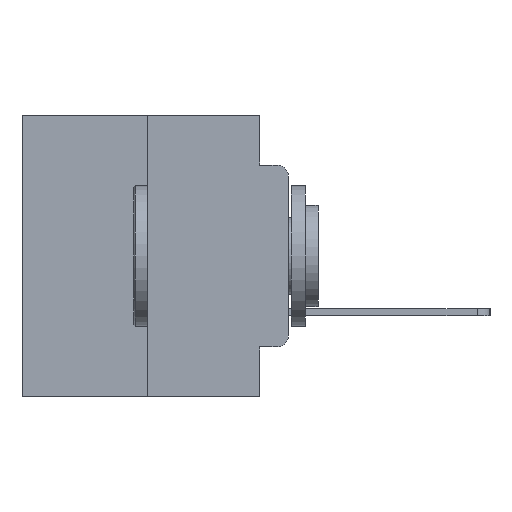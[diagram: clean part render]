
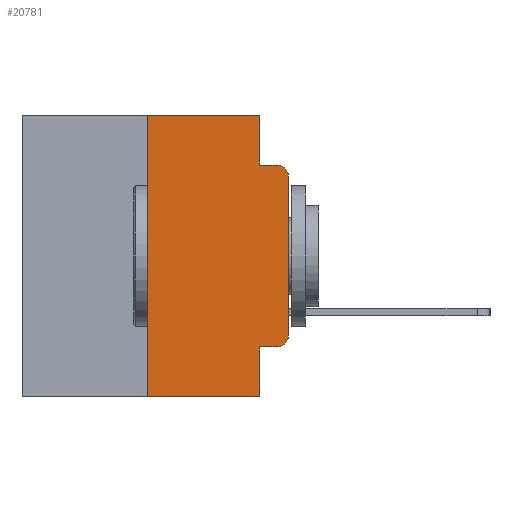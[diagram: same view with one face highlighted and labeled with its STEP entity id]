
A CAD part, left-side view. The second image highlights one B-rep face of the part: STEP entity #20781.
In plain terms, the highlighted planar face has unit normal (-1, 0, 0).
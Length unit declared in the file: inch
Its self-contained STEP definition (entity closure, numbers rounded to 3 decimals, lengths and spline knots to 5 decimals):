
#419 = EDGE_CURVE ( 'NONE', #8663, #21818, #3495, .T. ) ;
#1797 = ORIENTED_EDGE ( 'NONE', *, *, #419, .T. ) ;
#1842 = AXIS2_PLACEMENT_3D ( 'NONE', #24012, #11485, #26080 ) ;
#2052 = PLANE ( 'NONE',  #5337 ) ;
#2612 = VECTOR ( 'NONE', #22174, 39.37008 ) ;
#3182 = CARTESIAN_POINT ( 'NONE',  ( 0., 0.051, 0. ) ) ;
#3195 = CARTESIAN_POINT ( 'NONE',  ( 0., 0.473, 0. ) ) ;
#3435 = VERTEX_POINT ( 'NONE', #15398 ) ;
#3495 = LINE ( 'NONE', #5532, #24544 ) ;
#3558 = EDGE_CURVE ( 'NONE', #20752, #16808, #25629, .T. ) ;
#3563 = CARTESIAN_POINT ( 'NONE',  ( 0., 0.25, -0.5 ) ) ;
#3570 = CIRCLE ( 'NONE', #1842, 0.02 ) ;
#3607 = LINE ( 'NONE', #26743, #25941 ) ;
#3719 = EDGE_CURVE ( 'NONE', #14574, #13075, #3607, .T. ) ;
#3891 = ORIENTED_EDGE ( 'NONE', *, *, #3558, .F. ) ;
#4219 = ORIENTED_EDGE ( 'NONE', *, *, #25009, .F. ) ;
#4962 = VECTOR ( 'NONE', #10545, 39.37008 ) ;
#5025 = DIRECTION ( 'NONE',  ( 0., 0., -1. ) ) ;
#5337 = AXIS2_PLACEMENT_3D ( 'NONE', #10537, #25245, #12712 ) ;
#5505 = VECTOR ( 'NONE', #20684, 39.37008 ) ;
#5532 = CARTESIAN_POINT ( 'NONE',  ( 0., 0., 0. ) ) ;
#6277 = CARTESIAN_POINT ( 'NONE',  ( 0., 0.051, -0.0885 ) ) ;
#6573 = ORIENTED_EDGE ( 'NONE', *, *, #3719, .T. ) ;
#7925 = ORIENTED_EDGE ( 'NONE', *, *, #10982, .T. ) ;
#8055 = LINE ( 'NONE', #13450, #12942 ) ;
#8663 = VERTEX_POINT ( 'NONE', #10438 ) ;
#8932 = CIRCLE ( 'NONE', #16499, 0.02 ) ;
#8959 = DIRECTION ( 'NONE',  ( 0., 0., -1. ) ) ;
#9341 = LINE ( 'NONE', #19435, #14285 ) ;
#9593 = EDGE_CURVE ( 'NONE', #3435, #8663, #8932, .T. ) ;
#9643 = CARTESIAN_POINT ( 'NONE',  ( 0., 0.051, -0.0885 ) ) ;
#9742 = LINE ( 'NONE', #13817, #20249 ) ;
#9857 = CARTESIAN_POINT ( 'NONE',  ( 0., 0.02, -0.3915 ) ) ;
#10438 = CARTESIAN_POINT ( 'NONE',  ( 0., 0., -0.3915 ) ) ;
#10537 = CARTESIAN_POINT ( 'NONE',  ( 0., 0.473, 0. ) ) ;
#10545 = DIRECTION ( 'NONE',  ( 0., -1., 0. ) ) ;
#10982 = EDGE_CURVE ( 'NONE', #21681, #3435, #11123, .T. ) ;
#11123 = LINE ( 'NONE', #12231, #5505 ) ;
#11267 = LINE ( 'NONE', #6277, #4962 ) ;
#11485 = DIRECTION ( 'NONE',  ( -1., 0., 0. ) ) ;
#11933 = DIRECTION ( 'NONE',  ( 0., 0., -1. ) ) ;
#12160 = DIRECTION ( 'NONE',  ( 0., -1., 0. ) ) ;
#12231 = CARTESIAN_POINT ( 'NONE',  ( 0., 0.051, -0.4115 ) ) ;
#12712 = DIRECTION ( 'NONE',  ( 0., 0., -1. ) ) ;
#12942 = VECTOR ( 'NONE', #5025, 39.37008 ) ;
#13075 = VERTEX_POINT ( 'NONE', #21981 ) ;
#13450 = CARTESIAN_POINT ( 'NONE',  ( 0., 0.051, 0. ) ) ;
#13817 = CARTESIAN_POINT ( 'NONE',  ( 0., 0.25, 0. ) ) ;
#14285 = VECTOR ( 'NONE', #8959, 39.37008 ) ;
#14574 = VERTEX_POINT ( 'NONE', #3563 ) ;
#15398 = CARTESIAN_POINT ( 'NONE',  ( 0., 0.02, -0.4115 ) ) ;
#15904 = DIRECTION ( 'NONE',  ( 0., 0., 1. ) ) ;
#15987 = CARTESIAN_POINT ( 'NONE',  ( 0., 0.051, -0.4115 ) ) ;
#16499 = AXIS2_PLACEMENT_3D ( 'NONE', #9857, #24488, #11933 ) ;
#16629 = EDGE_CURVE ( 'NONE', #21681, #13075, #9341, .T. ) ;
#16775 = CARTESIAN_POINT ( 'NONE',  ( 0., 0.25, 0. ) ) ;
#16808 = VERTEX_POINT ( 'NONE', #3182 ) ;
#17784 = ORIENTED_EDGE ( 'NONE', *, *, #16629, .F. ) ;
#18062 = EDGE_CURVE ( 'NONE', #14574, #20752, #9742, .T. ) ;
#18343 = VERTEX_POINT ( 'NONE', #25200 ) ;
#18557 = CARTESIAN_POINT ( 'NONE',  ( 0., 0., -0.1085 ) ) ;
#18665 = VERTEX_POINT ( 'NONE', #9643 ) ;
#18755 = ORIENTED_EDGE ( 'NONE', *, *, #19456, .F. ) ;
#18963 = FACE_OUTER_BOUND ( 'NONE', #21901, .T. ) ;
#19435 = CARTESIAN_POINT ( 'NONE',  ( 0., 0.051, 0. ) ) ;
#19456 = EDGE_CURVE ( 'NONE', #16808, #18665, #8055, .T. ) ;
#20016 = ORIENTED_EDGE ( 'NONE', *, *, #26369, .T. ) ;
#20249 = VECTOR ( 'NONE', #15904, 39.37008 ) ;
#20410 = ORIENTED_EDGE ( 'NONE', *, *, #9593, .T. ) ;
#20684 = DIRECTION ( 'NONE',  ( 0., -1., 0. ) ) ;
#20719 = ORIENTED_EDGE ( 'NONE', *, *, #18062, .F. ) ;
#20752 = VERTEX_POINT ( 'NONE', #16775 ) ;
#20781 = ADVANCED_FACE ( 'NONE', ( #18963 ), #2052, .F. ) ;
#21681 = VERTEX_POINT ( 'NONE', #15987 ) ;
#21818 = VERTEX_POINT ( 'NONE', #18557 ) ;
#21901 = EDGE_LOOP ( 'NONE', ( #1797, #20016, #4219, #18755, #3891, #20719, #6573, #17784, #7925, #20410 ) ) ;
#21981 = CARTESIAN_POINT ( 'NONE',  ( 0., 0.051, -0.5 ) ) ;
#22174 = DIRECTION ( 'NONE',  ( 0., -1., 0. ) ) ;
#24012 = CARTESIAN_POINT ( 'NONE',  ( 0., 0.02, -0.1085 ) ) ;
#24448 = DIRECTION ( 'NONE',  ( 0., 0., 1. ) ) ;
#24488 = DIRECTION ( 'NONE',  ( -1., 0., 0. ) ) ;
#24544 = VECTOR ( 'NONE', #24448, 39.37008 ) ;
#25009 = EDGE_CURVE ( 'NONE', #18665, #18343, #11267, .T. ) ;
#25200 = CARTESIAN_POINT ( 'NONE',  ( 0., 0.02, -0.0885 ) ) ;
#25245 = DIRECTION ( 'NONE',  ( 1., 0., 0. ) ) ;
#25629 = LINE ( 'NONE', #3195, #2612 ) ;
#25941 = VECTOR ( 'NONE', #12160, 39.37008 ) ;
#26080 = DIRECTION ( 'NONE',  ( 0., 0., -1. ) ) ;
#26369 = EDGE_CURVE ( 'NONE', #21818, #18343, #3570, .T. ) ;
#26743 = CARTESIAN_POINT ( 'NONE',  ( 0., 0.473, -0.5 ) ) ;
